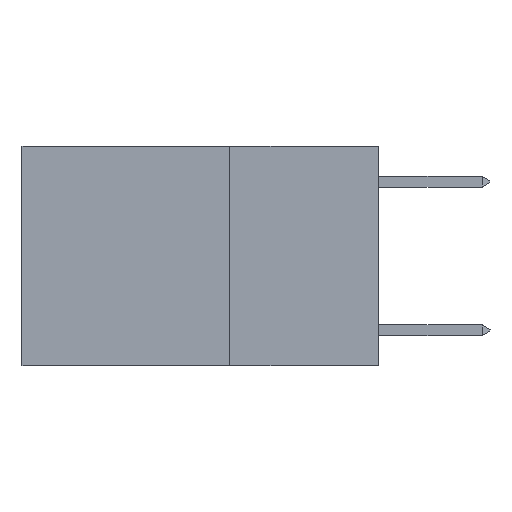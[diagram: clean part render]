
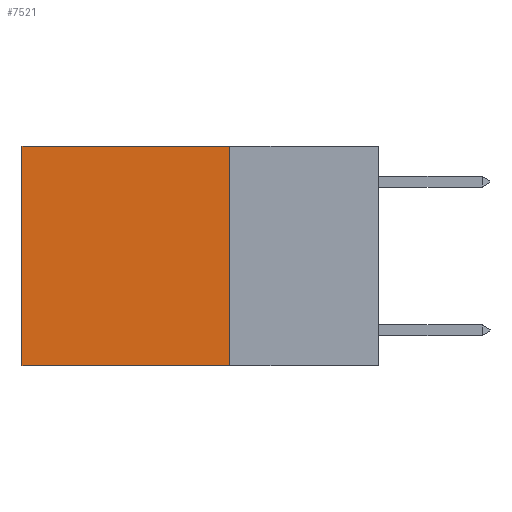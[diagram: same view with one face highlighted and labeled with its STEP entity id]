
A CAD part, left-side view. The second image highlights one B-rep face of the part: STEP entity #7521.
In plain terms, the highlighted planar face has unit normal (-1, 0, 0).
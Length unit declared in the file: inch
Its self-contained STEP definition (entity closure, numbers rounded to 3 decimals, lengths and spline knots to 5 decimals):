
#855 = PLANE ( 'NONE',  #8776 ) ;
#1020 = EDGE_LOOP ( 'NONE', ( #26224, #13665, #13141, #6162 ) ) ;
#1022 = VECTOR ( 'NONE', #2405, 39.37008 ) ;
#1512 = EDGE_CURVE ( 'NONE', #15507, #7450, #6987, .T. ) ;
#1870 = DIRECTION ( 'NONE',  ( 0., 0., -1. ) ) ;
#2108 = FACE_OUTER_BOUND ( 'NONE', #1020, .T. ) ;
#2405 = DIRECTION ( 'NONE',  ( 0., 0., -1. ) ) ;
#4427 = EDGE_CURVE ( 'NONE', #21463, #6724, #31707, .T. ) ;
#6111 = CARTESIAN_POINT ( 'NONE',  ( 0.2625, 0.25, 0. ) ) ;
#6162 = ORIENTED_EDGE ( 'NONE', *, *, #4427, .T. ) ;
#6724 = VERTEX_POINT ( 'NONE', #31233 ) ;
#6743 = VECTOR ( 'NONE', #28462, 39.37008 ) ;
#6947 = LINE ( 'NONE', #14736, #14591 ) ;
#6987 = LINE ( 'NONE', #22905, #6743 ) ;
#7450 = VERTEX_POINT ( 'NONE', #11038 ) ;
#7521 = ADVANCED_FACE ( 'NONE', ( #2108 ), #855, .F. ) ;
#7533 = CARTESIAN_POINT ( 'NONE',  ( 0.2625, 0.25, 0. ) ) ;
#8776 = AXIS2_PLACEMENT_3D ( 'NONE', #6111, #29039, #13847 ) ;
#11038 = CARTESIAN_POINT ( 'NONE',  ( 0.2625, 0.6, -0.37 ) ) ;
#11860 = EDGE_CURVE ( 'NONE', #21463, #15507, #6947, .T. ) ;
#11976 = CARTESIAN_POINT ( 'NONE',  ( 0.2625, 0.25, 0. ) ) ;
#13141 = ORIENTED_EDGE ( 'NONE', *, *, #11860, .F. ) ;
#13540 = CARTESIAN_POINT ( 'NONE',  ( 0.2625, 0.25, -0.37 ) ) ;
#13665 = ORIENTED_EDGE ( 'NONE', *, *, #1512, .F. ) ;
#13847 = DIRECTION ( 'NONE',  ( 0., 0., -1. ) ) ;
#14591 = VECTOR ( 'NONE', #1870, 39.37008 ) ;
#14736 = CARTESIAN_POINT ( 'NONE',  ( 0.2625, 0.25, 0. ) ) ;
#15257 = DIRECTION ( 'NONE',  ( 0., 1., 0. ) ) ;
#15507 = VERTEX_POINT ( 'NONE', #13540 ) ;
#21463 = VERTEX_POINT ( 'NONE', #11976 ) ;
#21606 = LINE ( 'NONE', #25416, #1022 ) ;
#22905 = CARTESIAN_POINT ( 'NONE',  ( 0.2625, 0.25, -0.37 ) ) ;
#22977 = EDGE_CURVE ( 'NONE', #6724, #7450, #21606, .T. ) ;
#25416 = CARTESIAN_POINT ( 'NONE',  ( 0.2625, 0.6, 0. ) ) ;
#26224 = ORIENTED_EDGE ( 'NONE', *, *, #22977, .T. ) ;
#28462 = DIRECTION ( 'NONE',  ( 0., 1., 0. ) ) ;
#29039 = DIRECTION ( 'NONE',  ( 1., 0., 0. ) ) ;
#31233 = CARTESIAN_POINT ( 'NONE',  ( 0.2625, 0.6, 0. ) ) ;
#31369 = VECTOR ( 'NONE', #15257, 39.37008 ) ;
#31707 = LINE ( 'NONE', #7533, #31369 ) ;
